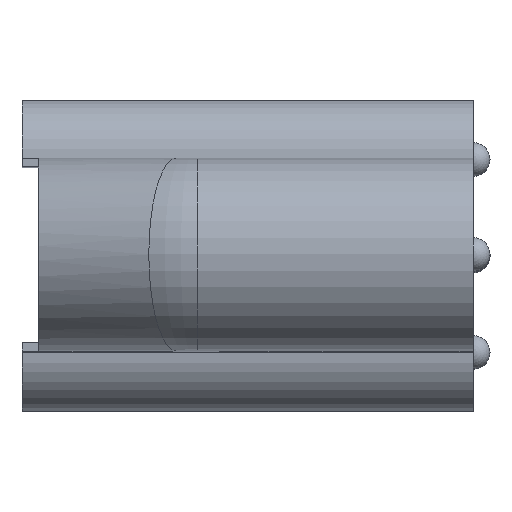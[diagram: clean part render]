
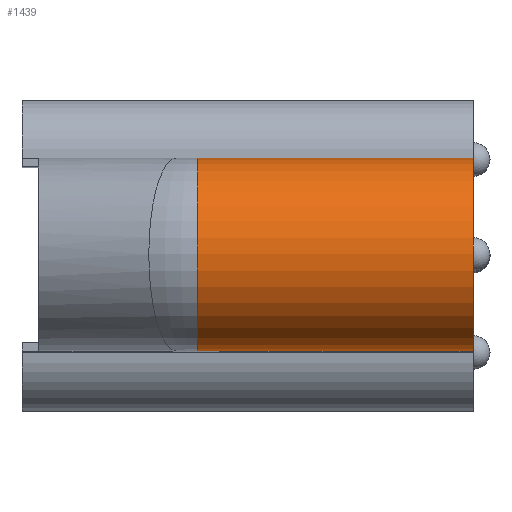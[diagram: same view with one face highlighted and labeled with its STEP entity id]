
A CAD part, top view. The second image highlights one B-rep face of the part: STEP entity #1439.
In plain terms, the highlighted cylindrical face has radius 11.509 mm (diameter 23.019 mm), a partial arc.
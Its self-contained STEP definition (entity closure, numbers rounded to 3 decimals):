
#62 = EDGE_CURVE ( 'NONE', #860, #1289, #1946, .T. ) ;
#85 = VERTEX_POINT ( 'NONE', #2524 ) ;
#105 = ORIENTED_EDGE ( 'NONE', *, *, #1955, .T. ) ;
#124 = DIRECTION ( 'NONE',  ( 1., 0., 0. ) ) ;
#216 = ORIENTED_EDGE ( 'NONE', *, *, #979, .F. ) ;
#232 = LINE ( 'NONE', #2529, #1959 ) ;
#342 = VERTEX_POINT ( 'NONE', #2256 ) ;
#397 = DIRECTION ( 'NONE',  ( -1., 0., 0. ) ) ;
#516 = CARTESIAN_POINT ( 'NONE',  ( 8.61, -25.532, 58.974 ) ) ;
#609 = DIRECTION ( 'NONE',  ( 0., 1., 0. ) ) ;
#807 = CIRCLE ( 'NONE', #2207, 11.509 ) ;
#860 = VERTEX_POINT ( 'NONE', #1308 ) ;
#891 = CYLINDRICAL_SURFACE ( 'NONE', #2062, 11.509 ) ;
#937 = DIRECTION ( 'NONE',  ( -1., 0., 0. ) ) ;
#958 = EDGE_CURVE ( 'NONE', #342, #1289, #807, .T. ) ;
#979 = EDGE_CURVE ( 'NONE', #342, #85, #232, .T. ) ;
#1033 = DIRECTION ( 'NONE',  ( 0., 1., 0. ) ) ;
#1199 = CIRCLE ( 'NONE', #2111, 11.509 ) ;
#1289 = VERTEX_POINT ( 'NONE', #2541 ) ;
#1308 = CARTESIAN_POINT ( 'NONE',  ( 8.61, -25.532, 58.974 ) ) ;
#1328 = VECTOR ( 'NONE', #937, 1000. ) ;
#1439 = ADVANCED_FACE ( 'NONE', ( #2450 ), #891, .T. ) ;
#1567 = CARTESIAN_POINT ( 'NONE',  ( -24.311, -14.022, 58.974 ) ) ;
#1846 = CARTESIAN_POINT ( 'NONE',  ( 12.729, -14.022, 58.974 ) ) ;
#1853 = EDGE_LOOP ( 'NONE', ( #2485, #105, #216, #2533 ) ) ;
#1946 = LINE ( 'NONE', #516, #1328 ) ;
#1955 = EDGE_CURVE ( 'NONE', #860, #85, #1199, .T. ) ;
#1959 = VECTOR ( 'NONE', #2341, 1000. ) ;
#1964 = DIRECTION ( 'NONE',  ( 0., 0., -1. ) ) ;
#2062 = AXIS2_PLACEMENT_3D ( 'NONE', #1846, #124, #1033 ) ;
#2111 = AXIS2_PLACEMENT_3D ( 'NONE', #2157, #397, #1964 ) ;
#2142 = DIRECTION ( 'NONE',  ( 1., 0., 0. ) ) ;
#2157 = CARTESIAN_POINT ( 'NONE',  ( 8.61, -14.022, 58.974 ) ) ;
#2207 = AXIS2_PLACEMENT_3D ( 'NONE', #1567, #2142, #609 ) ;
#2256 = CARTESIAN_POINT ( 'NONE',  ( -24.311, -2.513, 58.974 ) ) ;
#2341 = DIRECTION ( 'NONE',  ( 1., 0., 0. ) ) ;
#2450 = FACE_OUTER_BOUND ( 'NONE', #1853, .T. ) ;
#2485 = ORIENTED_EDGE ( 'NONE', *, *, #62, .F. ) ;
#2524 = CARTESIAN_POINT ( 'NONE',  ( 8.61, -2.513, 58.974 ) ) ;
#2529 = CARTESIAN_POINT ( 'NONE',  ( -24.311, -2.513, 58.974 ) ) ;
#2533 = ORIENTED_EDGE ( 'NONE', *, *, #958, .T. ) ;
#2541 = CARTESIAN_POINT ( 'NONE',  ( -24.311, -25.532, 58.974 ) ) ;
